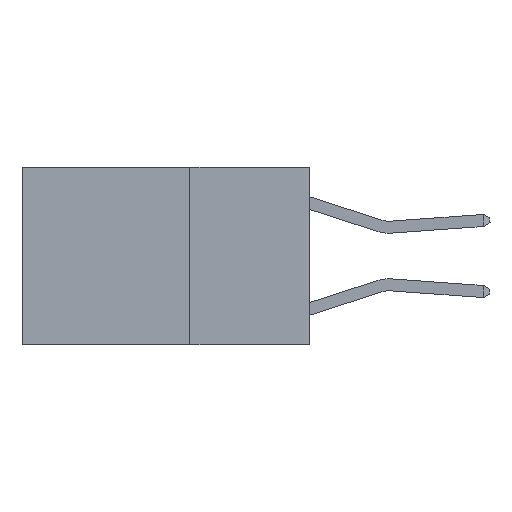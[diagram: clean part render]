
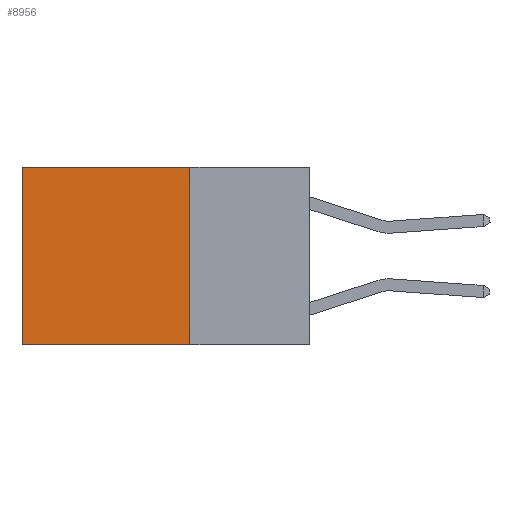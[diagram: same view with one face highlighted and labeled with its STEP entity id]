
A CAD part, left-side view. The second image highlights one B-rep face of the part: STEP entity #8956.
In plain terms, the highlighted planar face has unit normal (-1, 0, 0).
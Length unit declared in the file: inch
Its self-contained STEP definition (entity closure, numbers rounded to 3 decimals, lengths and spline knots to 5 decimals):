
#468 = ORIENTED_EDGE ( 'NONE', *, *, #4894, .T. ) ;
#690 = CARTESIAN_POINT ( 'NONE',  ( 0.2625, 0.25, 0. ) ) ;
#1365 = DIRECTION ( 'NONE',  ( 1., 0., 0. ) ) ;
#3951 = VERTEX_POINT ( 'NONE', #25397 ) ;
#4894 = EDGE_CURVE ( 'NONE', #3951, #12305, #19632, .T. ) ;
#6096 = PLANE ( 'NONE',  #7582 ) ;
#7582 = AXIS2_PLACEMENT_3D ( 'NONE', #7914, #1365, #22764 ) ;
#7814 = CARTESIAN_POINT ( 'NONE',  ( 0.2625, 0.25, -0.37 ) ) ;
#7914 = CARTESIAN_POINT ( 'NONE',  ( 0.2625, 0.25, 0. ) ) ;
#8111 = EDGE_CURVE ( 'NONE', #22838, #12305, #12107, .T. ) ;
#8298 = CARTESIAN_POINT ( 'NONE',  ( 0.2625, 0.25, 0. ) ) ;
#8343 = EDGE_LOOP ( 'NONE', ( #468, #23264, #23052, #20495 ) ) ;
#8715 = DIRECTION ( 'NONE',  ( 0., 0., -1. ) ) ;
#8956 = ADVANCED_FACE ( 'NONE', ( #24715 ), #6096, .F. ) ;
#11581 = VECTOR ( 'NONE', #24612, 39.37008 ) ;
#12107 = LINE ( 'NONE', #7814, #11581 ) ;
#12139 = CARTESIAN_POINT ( 'NONE',  ( 0.2625, 0.25, 0. ) ) ;
#12305 = VERTEX_POINT ( 'NONE', #12671 ) ;
#12671 = CARTESIAN_POINT ( 'NONE',  ( 0.2625, 0.6, -0.37 ) ) ;
#13128 = DIRECTION ( 'NONE',  ( 0., 0., -1. ) ) ;
#14466 = CARTESIAN_POINT ( 'NONE',  ( 0.2625, 0.25, -0.37 ) ) ;
#14548 = LINE ( 'NONE', #8298, #23694 ) ;
#15066 = CARTESIAN_POINT ( 'NONE',  ( 0.2625, 0.6, 0. ) ) ;
#16304 = VERTEX_POINT ( 'NONE', #690 ) ;
#16306 = DIRECTION ( 'NONE',  ( 0., 1., 0. ) ) ;
#16776 = EDGE_CURVE ( 'NONE', #16304, #3951, #24641, .T. ) ;
#18166 = EDGE_CURVE ( 'NONE', #16304, #22838, #14548, .T. ) ;
#19632 = LINE ( 'NONE', #15066, #26499 ) ;
#20495 = ORIENTED_EDGE ( 'NONE', *, *, #16776, .T. ) ;
#22764 = DIRECTION ( 'NONE',  ( 0., 0., -1. ) ) ;
#22838 = VERTEX_POINT ( 'NONE', #14466 ) ;
#23052 = ORIENTED_EDGE ( 'NONE', *, *, #18166, .F. ) ;
#23264 = ORIENTED_EDGE ( 'NONE', *, *, #8111, .F. ) ;
#23694 = VECTOR ( 'NONE', #8715, 39.37008 ) ;
#23738 = VECTOR ( 'NONE', #16306, 39.37008 ) ;
#24612 = DIRECTION ( 'NONE',  ( 0., 1., 0. ) ) ;
#24641 = LINE ( 'NONE', #12139, #23738 ) ;
#24715 = FACE_OUTER_BOUND ( 'NONE', #8343, .T. ) ;
#25397 = CARTESIAN_POINT ( 'NONE',  ( 0.2625, 0.6, 0. ) ) ;
#26499 = VECTOR ( 'NONE', #13128, 39.37008 ) ;
